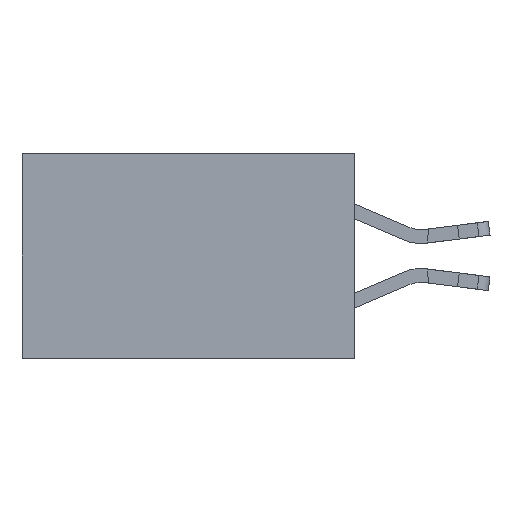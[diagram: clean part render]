
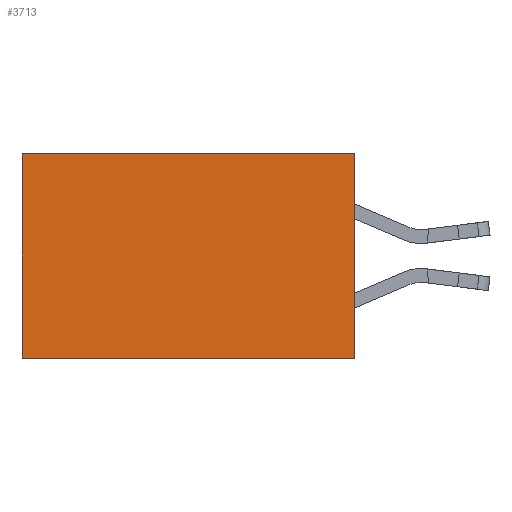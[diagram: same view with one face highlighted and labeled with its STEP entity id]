
A CAD part, left-side view. The second image highlights one B-rep face of the part: STEP entity #3713.
In plain terms, the highlighted planar face has unit normal (-1, 0, 0).
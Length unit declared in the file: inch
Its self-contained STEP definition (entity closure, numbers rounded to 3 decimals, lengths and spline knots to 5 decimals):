
#3539 = DIRECTION ( 'NONE',  ( 0., 0., -1. ) ) ;
#3713 = ADVANCED_FACE ( 'NONE', ( #16320 ), #7994, .F. ) ;
#5480 = CARTESIAN_POINT ( 'NONE',  ( 0.298, 0., 0. ) ) ;
#6988 = ORIENTED_EDGE ( 'NONE', *, *, #15103, .T. ) ;
#7516 = DIRECTION ( 'NONE',  ( 0., 1., 0. ) ) ;
#7994 = PLANE ( 'NONE',  #10139 ) ;
#9061 = VECTOR ( 'NONE', #3539, 39.37008 ) ;
#9422 = VECTOR ( 'NONE', #10333, 39.37008 ) ;
#9736 = EDGE_CURVE ( 'NONE', #18883, #25942, #22183, .T. ) ;
#9964 = CARTESIAN_POINT ( 'NONE',  ( 0.298, 0., -0.37 ) ) ;
#10139 = AXIS2_PLACEMENT_3D ( 'NONE', #5480, #15476, #14740 ) ;
#10333 = DIRECTION ( 'NONE',  ( 0., 0., -1. ) ) ;
#10964 = VERTEX_POINT ( 'NONE', #9964 ) ;
#11553 = DIRECTION ( 'NONE',  ( 0., 1., 0. ) ) ;
#12079 = ORIENTED_EDGE ( 'NONE', *, *, #23320, .F. ) ;
#13933 = CARTESIAN_POINT ( 'NONE',  ( 0.298, 0.6, -0.37 ) ) ;
#14740 = DIRECTION ( 'NONE',  ( 0., 0., -1. ) ) ;
#15103 = EDGE_CURVE ( 'NONE', #29973, #18883, #23640, .T. ) ;
#15476 = DIRECTION ( 'NONE',  ( 1., 0., 0. ) ) ;
#15800 = ORIENTED_EDGE ( 'NONE', *, *, #25695, .F. ) ;
#16320 = FACE_OUTER_BOUND ( 'NONE', #28889, .T. ) ;
#18883 = VERTEX_POINT ( 'NONE', #28340 ) ;
#21494 = CARTESIAN_POINT ( 'NONE',  ( 0.298, 0., 0. ) ) ;
#22183 = LINE ( 'NONE', #22226, #9061 ) ;
#22226 = CARTESIAN_POINT ( 'NONE',  ( 0.298, 0.6, 0. ) ) ;
#22529 = LINE ( 'NONE', #26530, #9422 ) ;
#22828 = CARTESIAN_POINT ( 'NONE',  ( 0.298, 0., 0. ) ) ;
#23320 = EDGE_CURVE ( 'NONE', #10964, #25942, #25447, .T. ) ;
#23640 = LINE ( 'NONE', #21494, #29632 ) ;
#24745 = VECTOR ( 'NONE', #11553, 39.37008 ) ;
#25447 = LINE ( 'NONE', #27590, #24745 ) ;
#25695 = EDGE_CURVE ( 'NONE', #29973, #10964, #22529, .T. ) ;
#25942 = VERTEX_POINT ( 'NONE', #13933 ) ;
#26530 = CARTESIAN_POINT ( 'NONE',  ( 0.298, 0., 0. ) ) ;
#27590 = CARTESIAN_POINT ( 'NONE',  ( 0.298, 0., -0.37 ) ) ;
#28340 = CARTESIAN_POINT ( 'NONE',  ( 0.298, 0.6, 0. ) ) ;
#28889 = EDGE_LOOP ( 'NONE', ( #29592, #12079, #15800, #6988 ) ) ;
#29592 = ORIENTED_EDGE ( 'NONE', *, *, #9736, .T. ) ;
#29632 = VECTOR ( 'NONE', #7516, 39.37008 ) ;
#29973 = VERTEX_POINT ( 'NONE', #22828 ) ;
